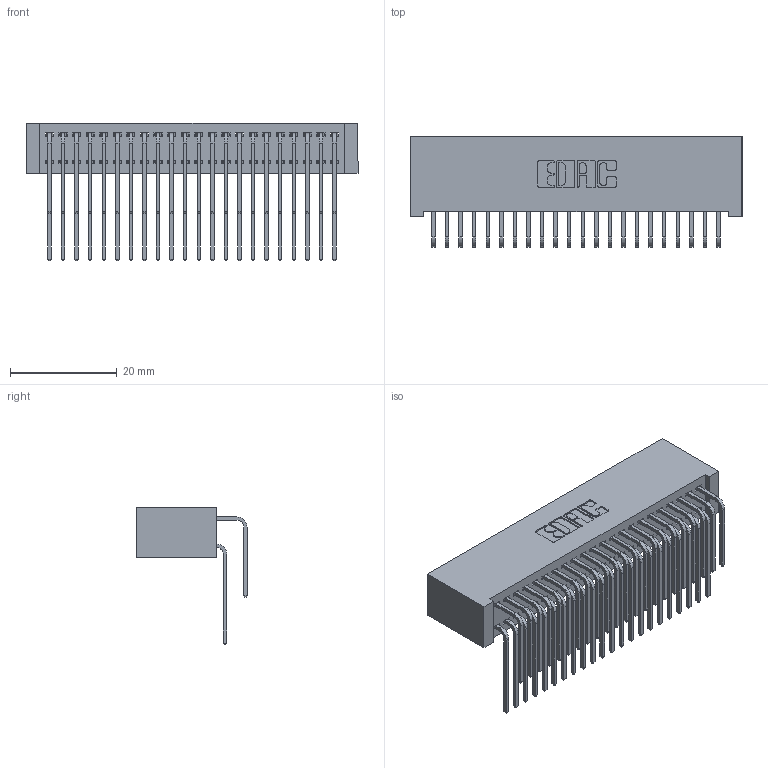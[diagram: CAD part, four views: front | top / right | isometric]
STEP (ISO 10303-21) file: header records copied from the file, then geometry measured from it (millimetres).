
FILE_DESCRIPTION (( 'STEP AP203' ), '1' );
FILE_NAME ('342-044-559-201.STEP', '2019-10-02T19:37:01', ( '' ), ( '' ), 'SwSTEP 2.0', 'SolidWorks 2016', '' );
FILE_SCHEMA (( 'CONFIG_CONTROL_DESIGN' ));
Length unit declared in the file: inch
Products named in the file (4): 342 Part_Lugless; 345-292-001_558 559 Tail - 1; 345-292-001_559 Tail - 2; 342-044-559-201
Assembly tree (45 placements, depth 2):
  342-044-559-201
    342 Part_Lugless
    345-292-001_558 559 Tail - 1  x22
    345-292-001_559 Tail - 2  x22
Bounding box: 62.13 x 20.64 x 25.78 mm (x, y, z)
Volume: 6180.9 mm3; surface area: 11162.6 mm2
Topology: 45 solids, 45 shells, 2478 faces, 7359 edges, 4846 vertices
Faces by surface type: plane 1734, cylinder 744
Entity records: 18115 total; most frequent: CARTESIAN_POINT 3073, ORIENTED_EDGE 2958, DIRECTION 2635, EDGE_CURVE 1479, LINE 1319, VECTOR 1319, VERTEX_POINT 982, AXIS2_PLACEMENT_3D 658
